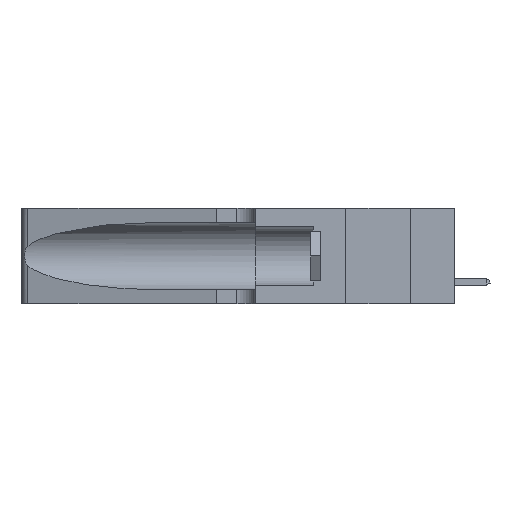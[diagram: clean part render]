
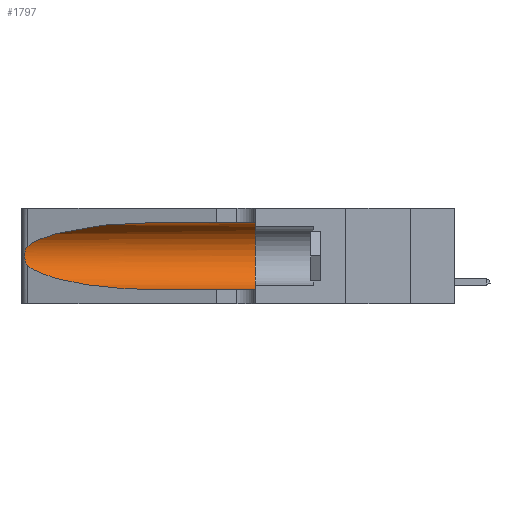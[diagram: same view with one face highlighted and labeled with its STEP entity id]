
A CAD part, left-side view. The second image highlights one B-rep face of the part: STEP entity #1797.
In plain terms, the highlighted cylindrical face has radius 3.308 mm (diameter 6.617 mm), a partial arc.
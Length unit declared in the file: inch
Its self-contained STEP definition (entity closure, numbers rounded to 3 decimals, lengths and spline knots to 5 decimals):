
#180 = EDGE_CURVE ( 'NONE', #3349, #7566, #2992, .T. ) ;
#291 = FACE_OUTER_BOUND ( 'NONE', #15899, .T. ) ;
#300 = CARTESIAN_POINT ( 'NONE',  ( 0.1305, 0.72297, 0.05475 ) ) ;
#699 = CARTESIAN_POINT ( 'NONE',  ( 0.18966, 0.96281, 0.05475 ) ) ;
#993 = VERTEX_POINT ( 'NONE', #17912 ) ;
#1396 = CARTESIAN_POINT ( 'NONE',  ( 0.25639, 1.23184, 0.21858 ) ) ;
#1797 = ADVANCED_FACE ( 'NONE', ( #291 ), #13007, .F. ) ;
#1813 = DIRECTION ( 'NONE',  ( 0., 0., 1. ) ) ;
#2007 = DIRECTION ( 'NONE',  ( 0., 1., 0. ) ) ;
#2241 = DIRECTION ( 'NONE',  ( 0., -1., 0. ) ) ;
#2563 = LINE ( 'NONE', #12203, #17961 ) ;
#2780 = EDGE_CURVE ( 'NONE', #9058, #993, #5209, .T. ) ;
#2867 = VERTEX_POINT ( 'NONE', #13049 ) ;
#2992 = LINE ( 'NONE', #5808, #7917 ) ;
#3349 = VERTEX_POINT ( 'NONE', #6632 ) ;
#3790 = DIRECTION ( 'NONE',  ( 0., 0., -1. ) ) ;
#4075 =( BOUNDED_CURVE ( )  B_SPLINE_CURVE ( 3, ( #4911, #16522, #4204, #4693 ),
 .UNSPECIFIED., .F., .F. ) 
 B_SPLINE_CURVE_WITH_KNOTS ( ( 4, 4 ),
 ( 1.5708, 2.84003 ),
 .UNSPECIFIED. ) 
 CURVE ( )  GEOMETRIC_REPRESENTATION_ITEM ( )  RATIONAL_B_SPLINE_CURVE ( ( 1., 0.87, 0.87, 1. ) ) 
 REPRESENTATION_ITEM ( '' )  );
#4204 = CARTESIAN_POINT ( 'NONE',  ( 0.2373, 1.15595, 0.28018 ) ) ;
#4243 = CARTESIAN_POINT ( 'NONE',  ( 0.25639, 1.23186, 0.15144 ) ) ;
#4357 = CARTESIAN_POINT ( 'NONE',  ( 0.26075, 1.23896, 0.19203 ) ) ;
#4693 = CARTESIAN_POINT ( 'NONE',  ( 0.25487, 1.22718, 0.22369 ) ) ;
#4872 = VERTEX_POINT ( 'NONE', #11973 ) ;
#4911 = CARTESIAN_POINT ( 'NONE',  ( 0.1305, 0.72297, 0.31525 ) ) ;
#5158 = CARTESIAN_POINT ( 'NONE',  ( 0.1305, 1.61858, 0.185 ) ) ;
#5209 = B_SPLINE_CURVE_WITH_KNOTS ( 'NONE', 3,
 ( #15477, #12739, #1396, #8560, #16975, #14360, #4357, #5683, #18362, #18476, #8380, #4243, #10054, #14120 ),
 .UNSPECIFIED., .F., .F.,
 ( 4, 2, 2, 2, 2, 2, 4 ),
 ( 0., 0.00027, 0.00053, 0.00107, 0.0016, 0.00187, 0.00214 ),
 .UNSPECIFIED. ) ;
#5210 = ORIENTED_EDGE ( 'NONE', *, *, #11213, .T. ) ;
#5340 = ORIENTED_EDGE ( 'NONE', *, *, #15835, .F. ) ;
#5683 = CARTESIAN_POINT ( 'NONE',  ( 0.26075, 1.23896, 0.178 ) ) ;
#5808 = CARTESIAN_POINT ( 'NONE',  ( 0.1305, 1.61858, 0.05475 ) ) ;
#6360 = CARTESIAN_POINT ( 'NONE',  ( 0.25487, 1.22718, 0.14631 ) ) ;
#6452 = AXIS2_PLACEMENT_3D ( 'NONE', #13232, #2007, #1813 ) ;
#6632 = CARTESIAN_POINT ( 'NONE',  ( 0.1305, 0.72297, 0.05475 ) ) ;
#6727 = ORIENTED_EDGE ( 'NONE', *, *, #2780, .T. ) ;
#7356 = CARTESIAN_POINT ( 'NONE',  ( 0.25487, 1.22718, 0.22369 ) ) ;
#7394 =( BOUNDED_CURVE ( )  B_SPLINE_CURVE ( 3, ( #6360, #12258, #699, #300 ),
 .UNSPECIFIED., .F., .F. ) 
 B_SPLINE_CURVE_WITH_KNOTS ( ( 4, 4 ),
 ( 3.44316, 4.71239 ),
 .UNSPECIFIED. ) 
 CURVE ( )  GEOMETRIC_REPRESENTATION_ITEM ( )  RATIONAL_B_SPLINE_CURVE ( ( 1., 0.87, 0.87, 1. ) ) 
 REPRESENTATION_ITEM ( '' )  );
#7566 = VERTEX_POINT ( 'NONE', #7648 ) ;
#7648 = CARTESIAN_POINT ( 'NONE',  ( 0.1305, 0.35, 0.05475 ) ) ;
#7917 = VECTOR ( 'NONE', #11525, 39.37008 ) ;
#8380 = CARTESIAN_POINT ( 'NONE',  ( 0.25789, 1.23486, 0.15765 ) ) ;
#8560 = CARTESIAN_POINT ( 'NONE',  ( 0.25787, 1.23484, 0.2124 ) ) ;
#8562 = AXIS2_PLACEMENT_3D ( 'NONE', #5158, #2241, #3790 ) ;
#9058 = VERTEX_POINT ( 'NONE', #7356 ) ;
#9840 = EDGE_CURVE ( 'NONE', #993, #3349, #7394, .T. ) ;
#10054 = CARTESIAN_POINT ( 'NONE',  ( 0.25555, 1.22993, 0.14849 ) ) ;
#10685 = EDGE_CURVE ( 'NONE', #2867, #7566, #15675, .T. ) ;
#11213 = EDGE_CURVE ( 'NONE', #4872, #9058, #4075, .T. ) ;
#11525 = DIRECTION ( 'NONE',  ( 0., -1., 0. ) ) ;
#11579 = ORIENTED_EDGE ( 'NONE', *, *, #180, .T. ) ;
#11973 = CARTESIAN_POINT ( 'NONE',  ( 0.1305, 0.72297, 0.31525 ) ) ;
#12203 = CARTESIAN_POINT ( 'NONE',  ( 0.1305, 1.61858, 0.31525 ) ) ;
#12258 = CARTESIAN_POINT ( 'NONE',  ( 0.2373, 1.15595, 0.08982 ) ) ;
#12739 = CARTESIAN_POINT ( 'NONE',  ( 0.25555, 1.22994, 0.2215 ) ) ;
#13007 = CYLINDRICAL_SURFACE ( 'NONE', #8562, 0.13025 ) ;
#13049 = CARTESIAN_POINT ( 'NONE',  ( 0.1305, 0.35, 0.31525 ) ) ;
#13232 = CARTESIAN_POINT ( 'NONE',  ( 0.1305, 0.35, 0.185 ) ) ;
#14120 = CARTESIAN_POINT ( 'NONE',  ( 0.25487, 1.22718, 0.14631 ) ) ;
#14360 = CARTESIAN_POINT ( 'NONE',  ( 0.26018, 1.23835, 0.19895 ) ) ;
#15023 = DIRECTION ( 'NONE',  ( 0., -1., 0. ) ) ;
#15477 = CARTESIAN_POINT ( 'NONE',  ( 0.25487, 1.22718, 0.22369 ) ) ;
#15675 = CIRCLE ( 'NONE', #6452, 0.13025 ) ;
#15835 = EDGE_CURVE ( 'NONE', #4872, #2867, #2563, .T. ) ;
#15899 = EDGE_LOOP ( 'NONE', ( #5210, #6727, #16667, #11579, #17943, #5340 ) ) ;
#16522 = CARTESIAN_POINT ( 'NONE',  ( 0.18966, 0.96281, 0.31525 ) ) ;
#16667 = ORIENTED_EDGE ( 'NONE', *, *, #9840, .T. ) ;
#16975 = CARTESIAN_POINT ( 'NONE',  ( 0.25854, 1.2359, 0.20912 ) ) ;
#17912 = CARTESIAN_POINT ( 'NONE',  ( 0.25487, 1.22718, 0.14631 ) ) ;
#17943 = ORIENTED_EDGE ( 'NONE', *, *, #10685, .F. ) ;
#17961 = VECTOR ( 'NONE', #15023, 39.37008 ) ;
#18362 = CARTESIAN_POINT ( 'NONE',  ( 0.26017, 1.23833, 0.17102 ) ) ;
#18476 = CARTESIAN_POINT ( 'NONE',  ( 0.25856, 1.23593, 0.16098 ) ) ;
